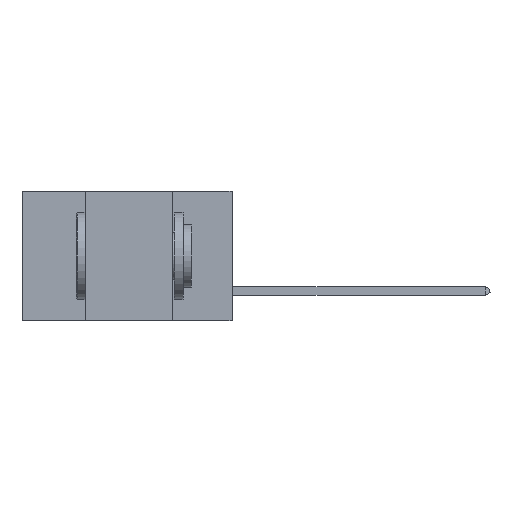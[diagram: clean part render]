
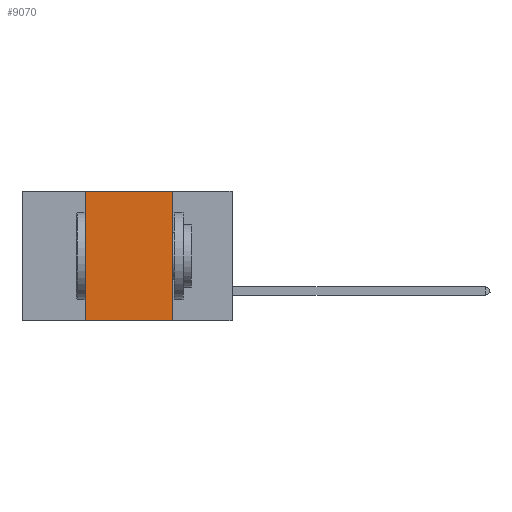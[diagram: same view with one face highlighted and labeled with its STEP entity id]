
A CAD part, left-side view. The second image highlights one B-rep face of the part: STEP entity #9070.
In plain terms, the highlighted planar face has unit normal (-1, 0, 0).
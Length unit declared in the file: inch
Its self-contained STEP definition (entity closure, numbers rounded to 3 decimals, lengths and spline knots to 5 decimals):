
#945 = DIRECTION ( 'NONE',  ( 0., 0., -1. ) ) ;
#1887 = LINE ( 'NONE', #18111, #18512 ) ;
#4250 = LINE ( 'NONE', #27571, #6846 ) ;
#5807 = ORIENTED_EDGE ( 'NONE', *, *, #18547, .T. ) ;
#5893 = DIRECTION ( 'NONE',  ( 1., 0., 0. ) ) ;
#6046 = AXIS2_PLACEMENT_3D ( 'NONE', #15332, #5893, #945 ) ;
#6846 = VECTOR ( 'NONE', #17948, 39.37008 ) ;
#9070 = ADVANCED_FACE ( 'NONE', ( #15601 ), #13061, .F. ) ;
#9634 = ORIENTED_EDGE ( 'NONE', *, *, #13329, .F. ) ;
#9774 = LINE ( 'NONE', #25643, #15744 ) ;
#10332 = ORIENTED_EDGE ( 'NONE', *, *, #21490, .F. ) ;
#11500 = DIRECTION ( 'NONE',  ( 0., 0., 1. ) ) ;
#11706 = VERTEX_POINT ( 'NONE', #21317 ) ;
#12747 = CARTESIAN_POINT ( 'NONE',  ( 0., 0.17, 0. ) ) ;
#13061 = PLANE ( 'NONE',  #6046 ) ;
#13329 = EDGE_CURVE ( 'NONE', #21811, #27206, #4250, .T. ) ;
#13946 = EDGE_LOOP ( 'NONE', ( #10332, #9634, #24474, #5807 ) ) ;
#14634 = LINE ( 'NONE', #22225, #17581 ) ;
#14797 = CARTESIAN_POINT ( 'NONE',  ( 0., 0.42, 0. ) ) ;
#15332 = CARTESIAN_POINT ( 'NONE',  ( 0., 0.6, 0. ) ) ;
#15601 = FACE_OUTER_BOUND ( 'NONE', #13946, .T. ) ;
#15744 = VECTOR ( 'NONE', #11500, 39.37008 ) ;
#17577 = CARTESIAN_POINT ( 'NONE',  ( 0., 0.42, -0.37 ) ) ;
#17581 = VECTOR ( 'NONE', #27284, 39.37008 ) ;
#17948 = DIRECTION ( 'NONE',  ( 0., -1., 0. ) ) ;
#18111 = CARTESIAN_POINT ( 'NONE',  ( 0., 0.17, 0. ) ) ;
#18512 = VECTOR ( 'NONE', #23039, 39.37008 ) ;
#18547 = EDGE_CURVE ( 'NONE', #27354, #11706, #14634, .T. ) ;
#18901 = EDGE_CURVE ( 'NONE', #27354, #21811, #9774, .T. ) ;
#21317 = CARTESIAN_POINT ( 'NONE',  ( 0., 0.17, -0.37 ) ) ;
#21490 = EDGE_CURVE ( 'NONE', #27206, #11706, #1887, .T. ) ;
#21811 = VERTEX_POINT ( 'NONE', #14797 ) ;
#22225 = CARTESIAN_POINT ( 'NONE',  ( 0., 0.6, -0.37 ) ) ;
#23039 = DIRECTION ( 'NONE',  ( 0., 0., -1. ) ) ;
#24474 = ORIENTED_EDGE ( 'NONE', *, *, #18901, .F. ) ;
#25643 = CARTESIAN_POINT ( 'NONE',  ( 0., 0.42, 0. ) ) ;
#27206 = VERTEX_POINT ( 'NONE', #12747 ) ;
#27284 = DIRECTION ( 'NONE',  ( 0., -1., 0. ) ) ;
#27354 = VERTEX_POINT ( 'NONE', #17577 ) ;
#27571 = CARTESIAN_POINT ( 'NONE',  ( 0., 0.6, 0. ) ) ;
